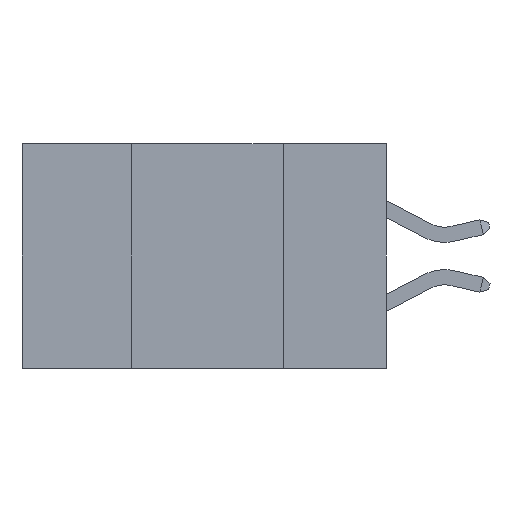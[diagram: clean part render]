
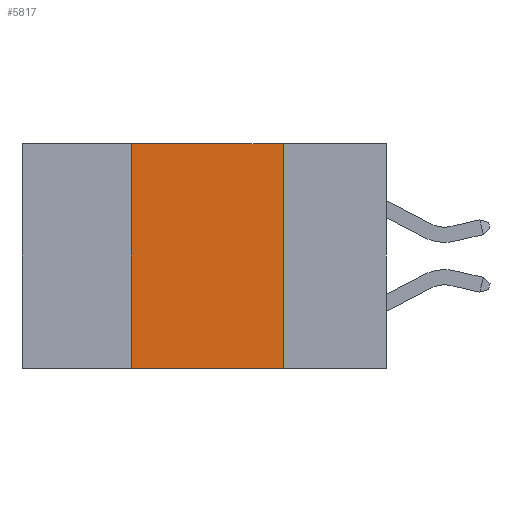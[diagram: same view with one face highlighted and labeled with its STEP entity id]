
A CAD part, left-side view. The second image highlights one B-rep face of the part: STEP entity #5817.
In plain terms, the highlighted planar face has unit normal (-1, 0, 0).
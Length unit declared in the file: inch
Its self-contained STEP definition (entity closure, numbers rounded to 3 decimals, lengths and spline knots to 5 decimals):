
#55 = DIRECTION ( 'NONE',  ( 0., -1., 0. ) ) ;
#297 = ORIENTED_EDGE ( 'NONE', *, *, #10828, .F. ) ;
#800 = DIRECTION ( 'NONE',  ( 1., 0., 0. ) ) ;
#989 = CARTESIAN_POINT ( 'NONE',  ( 0., 0.17, -0.37 ) ) ;
#1029 = CARTESIAN_POINT ( 'NONE',  ( 0., 0.42, -0.37 ) ) ;
#1409 = ORIENTED_EDGE ( 'NONE', *, *, #7604, .F. ) ;
#1749 = VERTEX_POINT ( 'NONE', #5065 ) ;
#1993 = ORIENTED_EDGE ( 'NONE', *, *, #10890, .T. ) ;
#2314 = FACE_OUTER_BOUND ( 'NONE', #7388, .T. ) ;
#2362 = VERTEX_POINT ( 'NONE', #10748 ) ;
#2692 = LINE ( 'NONE', #9121, #9368 ) ;
#3198 = ORIENTED_EDGE ( 'NONE', *, *, #7522, .F. ) ;
#3981 = CARTESIAN_POINT ( 'NONE',  ( 0., 0.6, -0.37 ) ) ;
#5065 = CARTESIAN_POINT ( 'NONE',  ( 0., 0.17, 0. ) ) ;
#5603 = AXIS2_PLACEMENT_3D ( 'NONE', #7011, #800, #7183 ) ;
#5817 = ADVANCED_FACE ( 'NONE', ( #2314 ), #7877, .F. ) ;
#5869 = VERTEX_POINT ( 'NONE', #9790 ) ;
#6022 = CARTESIAN_POINT ( 'NONE',  ( 0., 0.42, -0.37 ) ) ;
#6224 = VECTOR ( 'NONE', #9154, 39.37008 ) ;
#7011 = CARTESIAN_POINT ( 'NONE',  ( 0., 0.6, 0. ) ) ;
#7183 = DIRECTION ( 'NONE',  ( 0., 0., -1. ) ) ;
#7365 = DIRECTION ( 'NONE',  ( 0., 0., -1. ) ) ;
#7388 = EDGE_LOOP ( 'NONE', ( #3198, #1409, #297, #1993 ) ) ;
#7522 = EDGE_CURVE ( 'NONE', #1749, #2362, #9870, .T. ) ;
#7604 = EDGE_CURVE ( 'NONE', #5869, #1749, #2692, .T. ) ;
#7877 = PLANE ( 'NONE',  #5603 ) ;
#7904 = VECTOR ( 'NONE', #7365, 39.37008 ) ;
#8253 = DIRECTION ( 'NONE',  ( 0., 0., 1. ) ) ;
#8539 = LINE ( 'NONE', #3981, #6224 ) ;
#8549 = VERTEX_POINT ( 'NONE', #6022 ) ;
#9121 = CARTESIAN_POINT ( 'NONE',  ( 0., 0.6, 0. ) ) ;
#9154 = DIRECTION ( 'NONE',  ( 0., -1., 0. ) ) ;
#9368 = VECTOR ( 'NONE', #55, 39.37008 ) ;
#9790 = CARTESIAN_POINT ( 'NONE',  ( 0., 0.42, 0. ) ) ;
#9870 = LINE ( 'NONE', #989, #7904 ) ;
#10748 = CARTESIAN_POINT ( 'NONE',  ( 0., 0.17, -0.37 ) ) ;
#10828 = EDGE_CURVE ( 'NONE', #8549, #5869, #11192, .T. ) ;
#10890 = EDGE_CURVE ( 'NONE', #8549, #2362, #8539, .T. ) ;
#10941 = VECTOR ( 'NONE', #8253, 39.37008 ) ;
#11192 = LINE ( 'NONE', #1029, #10941 ) ;
